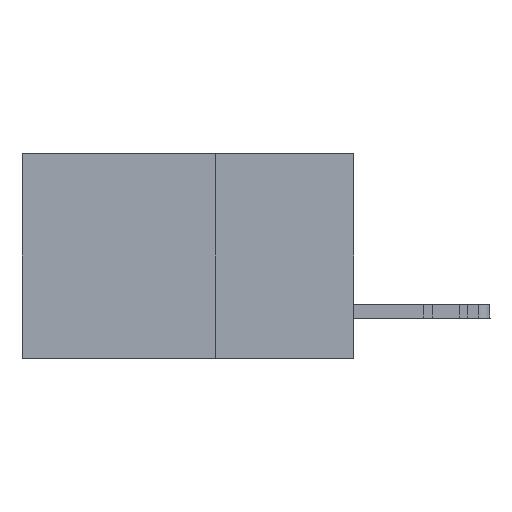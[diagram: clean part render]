
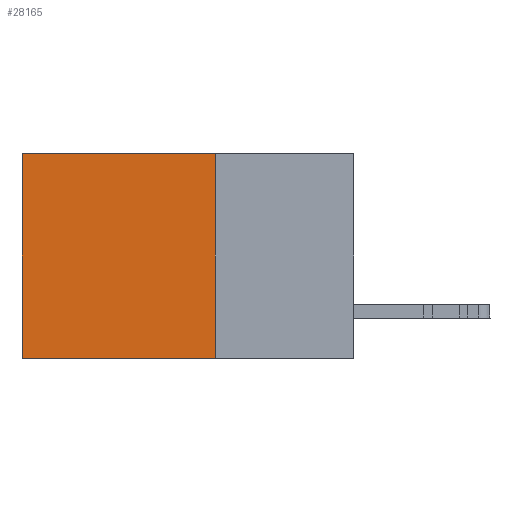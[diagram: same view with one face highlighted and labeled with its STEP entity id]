
A CAD part, left-side view. The second image highlights one B-rep face of the part: STEP entity #28165.
In plain terms, the highlighted planar face has unit normal (-1, 0, 0).
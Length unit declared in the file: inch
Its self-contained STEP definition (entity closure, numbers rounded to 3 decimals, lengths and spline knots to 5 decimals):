
#2352 = CARTESIAN_POINT ( 'NONE',  ( 0.2875, 0.25, -0.37 ) ) ;
#2604 = EDGE_CURVE ( 'NONE', #37236, #35173, #32130, .T. ) ;
#3828 = DIRECTION ( 'NONE',  ( 0., 0., -1. ) ) ;
#4017 = ORIENTED_EDGE ( 'NONE', *, *, #39800, .F. ) ;
#7353 = CARTESIAN_POINT ( 'NONE',  ( 0.2875, 0.25, -0.37 ) ) ;
#7513 = CARTESIAN_POINT ( 'NONE',  ( 0.2875, 0.25, 0. ) ) ;
#8085 = CARTESIAN_POINT ( 'NONE',  ( 0.2875, 0.6, -0.37 ) ) ;
#8182 = FACE_OUTER_BOUND ( 'NONE', #24264, .T. ) ;
#9764 = DIRECTION ( 'NONE',  ( 0., 0., -1. ) ) ;
#12490 = VERTEX_POINT ( 'NONE', #44872 ) ;
#13063 = CARTESIAN_POINT ( 'NONE',  ( 0.2875, 0.6, 0. ) ) ;
#13307 = PLANE ( 'NONE',  #36338 ) ;
#15375 = CARTESIAN_POINT ( 'NONE',  ( 0.2875, 0.25, 0. ) ) ;
#16202 = DIRECTION ( 'NONE',  ( 0., 1., 0. ) ) ;
#17781 = DIRECTION ( 'NONE',  ( 0., 1., 0. ) ) ;
#17851 = DIRECTION ( 'NONE',  ( 1., 0., 0. ) ) ;
#20864 = LINE ( 'NONE', #15375, #43694 ) ;
#20985 = CARTESIAN_POINT ( 'NONE',  ( 0.2875, 0.6, 0. ) ) ;
#24264 = EDGE_LOOP ( 'NONE', ( #42127, #30143, #4017, #44200 ) ) ;
#25029 = VECTOR ( 'NONE', #9764, 39.37008 ) ;
#25306 = EDGE_CURVE ( 'NONE', #42869, #35173, #45857, .T. ) ;
#27643 = VECTOR ( 'NONE', #17781, 39.37008 ) ;
#28165 = ADVANCED_FACE ( 'NONE', ( #8182 ), #13307, .F. ) ;
#30143 = ORIENTED_EDGE ( 'NONE', *, *, #2604, .F. ) ;
#32130 = LINE ( 'NONE', #2352, #41028 ) ;
#34187 = DIRECTION ( 'NONE',  ( 0., 0., -1. ) ) ;
#35084 = CARTESIAN_POINT ( 'NONE',  ( 0.2875, 0.25, 0. ) ) ;
#35173 = VERTEX_POINT ( 'NONE', #8085 ) ;
#36338 = AXIS2_PLACEMENT_3D ( 'NONE', #35084, #17851, #3828 ) ;
#37236 = VERTEX_POINT ( 'NONE', #7353 ) ;
#38503 = EDGE_CURVE ( 'NONE', #12490, #42869, #39424, .T. ) ;
#39424 = LINE ( 'NONE', #7513, #27643 ) ;
#39800 = EDGE_CURVE ( 'NONE', #12490, #37236, #20864, .T. ) ;
#41028 = VECTOR ( 'NONE', #16202, 39.37008 ) ;
#42127 = ORIENTED_EDGE ( 'NONE', *, *, #25306, .T. ) ;
#42869 = VERTEX_POINT ( 'NONE', #20985 ) ;
#43694 = VECTOR ( 'NONE', #34187, 39.37008 ) ;
#44200 = ORIENTED_EDGE ( 'NONE', *, *, #38503, .T. ) ;
#44872 = CARTESIAN_POINT ( 'NONE',  ( 0.2875, 0.25, 0. ) ) ;
#45857 = LINE ( 'NONE', #13063, #25029 ) ;
